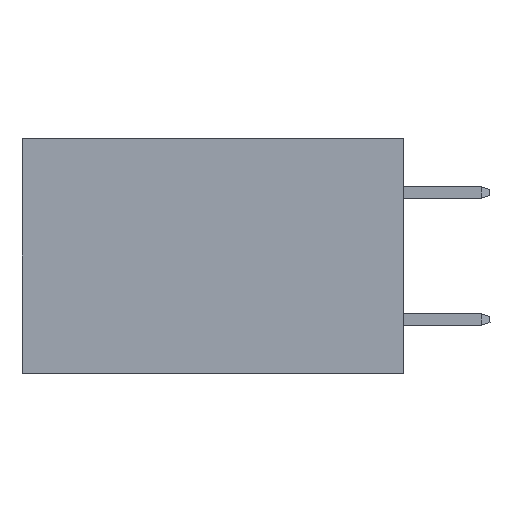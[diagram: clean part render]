
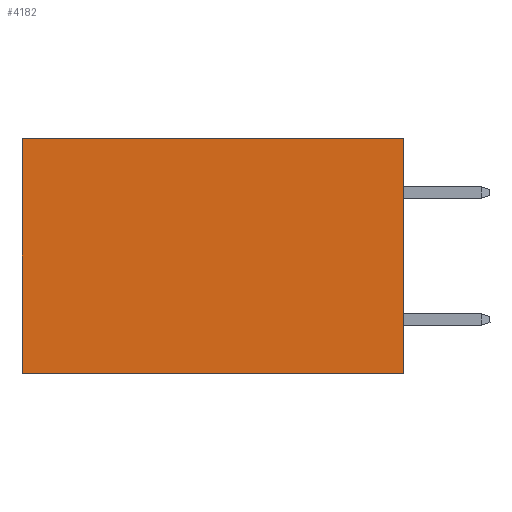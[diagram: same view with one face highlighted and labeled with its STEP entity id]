
A CAD part, left-side view. The second image highlights one B-rep face of the part: STEP entity #4182.
In plain terms, the highlighted planar face has unit normal (-1, 0, 0).
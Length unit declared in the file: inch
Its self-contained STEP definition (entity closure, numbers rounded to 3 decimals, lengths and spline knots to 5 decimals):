
#490 = EDGE_CURVE ( 'NONE', #9901, #1449, #7951, .T. ) ;
#662 = DIRECTION ( 'NONE',  ( 0., 0., -1. ) ) ;
#1449 = VERTEX_POINT ( 'NONE', #9421 ) ;
#2116 = VECTOR ( 'NONE', #9098, 39.37008 ) ;
#2201 = ORIENTED_EDGE ( 'NONE', *, *, #10215, .T. ) ;
#2658 = PLANE ( 'NONE',  #9988 ) ;
#4138 = CARTESIAN_POINT ( 'NONE',  ( 0.2875, 0., 0. ) ) ;
#4141 = LINE ( 'NONE', #7650, #8141 ) ;
#4182 = ADVANCED_FACE ( 'NONE', ( #10013 ), #2658, .F. ) ;
#4186 = CARTESIAN_POINT ( 'NONE',  ( 0.2875, 0., 0. ) ) ;
#4564 = VERTEX_POINT ( 'NONE', #8883 ) ;
#5136 = ORIENTED_EDGE ( 'NONE', *, *, #10265, .F. ) ;
#5422 = CARTESIAN_POINT ( 'NONE',  ( 0.2875, 0., 0. ) ) ;
#5426 = CARTESIAN_POINT ( 'NONE',  ( 0.2875, 0., 0. ) ) ;
#5839 = DIRECTION ( 'NONE',  ( 0., 1., 0. ) ) ;
#6008 = DIRECTION ( 'NONE',  ( 0., 1., 0. ) ) ;
#6371 = DIRECTION ( 'NONE',  ( 1., 0., 0. ) ) ;
#6387 = VECTOR ( 'NONE', #662, 39.37008 ) ;
#6469 = VECTOR ( 'NONE', #6008, 39.37008 ) ;
#7650 = CARTESIAN_POINT ( 'NONE',  ( 0.2875, 0., -0.37 ) ) ;
#7951 = LINE ( 'NONE', #4138, #6469 ) ;
#8141 = VECTOR ( 'NONE', #5839, 39.37008 ) ;
#8859 = ORIENTED_EDGE ( 'NONE', *, *, #10468, .F. ) ;
#8883 = CARTESIAN_POINT ( 'NONE',  ( 0.2875, 0., -0.37 ) ) ;
#9005 = CARTESIAN_POINT ( 'NONE',  ( 0.2875, 0.6, -0.37 ) ) ;
#9098 = DIRECTION ( 'NONE',  ( 0., 0., -1. ) ) ;
#9147 = DIRECTION ( 'NONE',  ( 0., 0., -1. ) ) ;
#9421 = CARTESIAN_POINT ( 'NONE',  ( 0.2875, 0.6, 0. ) ) ;
#9893 = LINE ( 'NONE', #9956, #2116 ) ;
#9901 = VERTEX_POINT ( 'NONE', #4186 ) ;
#9956 = CARTESIAN_POINT ( 'NONE',  ( 0.2875, 0.6, 0. ) ) ;
#9988 = AXIS2_PLACEMENT_3D ( 'NONE', #5422, #6371, #9147 ) ;
#10013 = FACE_OUTER_BOUND ( 'NONE', #10402, .T. ) ;
#10215 = EDGE_CURVE ( 'NONE', #1449, #11209, #9893, .T. ) ;
#10265 = EDGE_CURVE ( 'NONE', #9901, #4564, #11706, .T. ) ;
#10402 = EDGE_LOOP ( 'NONE', ( #2201, #8859, #5136, #11159 ) ) ;
#10468 = EDGE_CURVE ( 'NONE', #4564, #11209, #4141, .T. ) ;
#11159 = ORIENTED_EDGE ( 'NONE', *, *, #490, .T. ) ;
#11209 = VERTEX_POINT ( 'NONE', #9005 ) ;
#11706 = LINE ( 'NONE', #5426, #6387 ) ;
